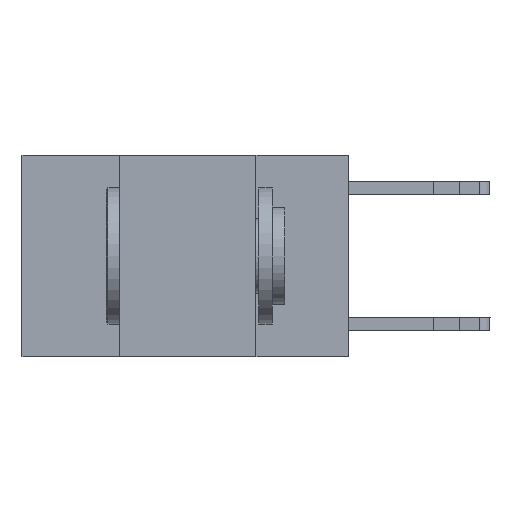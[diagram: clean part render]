
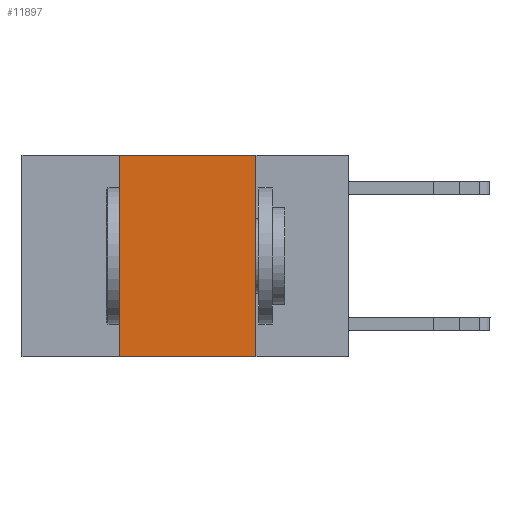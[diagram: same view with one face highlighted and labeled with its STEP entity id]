
A CAD part, left-side view. The second image highlights one B-rep face of the part: STEP entity #11897.
In plain terms, the highlighted planar face has unit normal (-1, 0, 0).
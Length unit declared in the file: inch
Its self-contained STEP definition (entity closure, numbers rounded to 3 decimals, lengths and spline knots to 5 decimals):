
#150 = CARTESIAN_POINT ( 'NONE',  ( 0., 0.42, -0.37 ) ) ;
#812 = CARTESIAN_POINT ( 'NONE',  ( 0., 0.17, 0. ) ) ;
#3263 = EDGE_CURVE ( 'NONE', #23601, #6398, #22165, .T. ) ;
#3587 = EDGE_LOOP ( 'NONE', ( #5036, #5144, #5211, #6932 ) ) ;
#4066 = VERTEX_POINT ( 'NONE', #9736 ) ;
#5036 = ORIENTED_EDGE ( 'NONE', *, *, #26090, .F. ) ;
#5144 = ORIENTED_EDGE ( 'NONE', *, *, #27211, .F. ) ;
#5211 = ORIENTED_EDGE ( 'NONE', *, *, #8322, .F. ) ;
#5277 = VECTOR ( 'NONE', #11252, 39.37008 ) ;
#5966 = LINE ( 'NONE', #6752, #5277 ) ;
#6398 = VERTEX_POINT ( 'NONE', #21103 ) ;
#6752 = CARTESIAN_POINT ( 'NONE',  ( 0., 0.17, 0. ) ) ;
#6932 = ORIENTED_EDGE ( 'NONE', *, *, #3263, .T. ) ;
#7623 = VERTEX_POINT ( 'NONE', #812 ) ;
#8322 = EDGE_CURVE ( 'NONE', #23601, #4066, #17761, .T. ) ;
#9736 = CARTESIAN_POINT ( 'NONE',  ( 0., 0.42, 0. ) ) ;
#11252 = DIRECTION ( 'NONE',  ( 0., 0., -1. ) ) ;
#11897 = ADVANCED_FACE ( 'NONE', ( #15045 ), #19527, .F. ) ;
#12204 = DIRECTION ( 'NONE',  ( 0., 0., 1. ) ) ;
#12390 = CARTESIAN_POINT ( 'NONE',  ( 0., 0.42, 0. ) ) ;
#15045 = FACE_OUTER_BOUND ( 'NONE', #3587, .T. ) ;
#15836 = LINE ( 'NONE', #17474, #20164 ) ;
#17474 = CARTESIAN_POINT ( 'NONE',  ( 0., 0.6, 0. ) ) ;
#17761 = LINE ( 'NONE', #12390, #17889 ) ;
#17873 = DIRECTION ( 'NONE',  ( 0., 0., -1. ) ) ;
#17889 = VECTOR ( 'NONE', #12204, 39.37008 ) ;
#18588 = VECTOR ( 'NONE', #23527, 39.37008 ) ;
#18877 = DIRECTION ( 'NONE',  ( 1., 0., 0. ) ) ;
#19527 = PLANE ( 'NONE',  #27577 ) ;
#19901 = CARTESIAN_POINT ( 'NONE',  ( 0., 0.6, 0. ) ) ;
#20164 = VECTOR ( 'NONE', #27967, 39.37008 ) ;
#21103 = CARTESIAN_POINT ( 'NONE',  ( 0., 0.17, -0.37 ) ) ;
#22165 = LINE ( 'NONE', #23426, #18588 ) ;
#23426 = CARTESIAN_POINT ( 'NONE',  ( 0., 0.6, -0.37 ) ) ;
#23527 = DIRECTION ( 'NONE',  ( 0., -1., 0. ) ) ;
#23601 = VERTEX_POINT ( 'NONE', #150 ) ;
#26090 = EDGE_CURVE ( 'NONE', #7623, #6398, #5966, .T. ) ;
#27211 = EDGE_CURVE ( 'NONE', #4066, #7623, #15836, .T. ) ;
#27577 = AXIS2_PLACEMENT_3D ( 'NONE', #19901, #18877, #17873 ) ;
#27967 = DIRECTION ( 'NONE',  ( 0., -1., 0. ) ) ;
